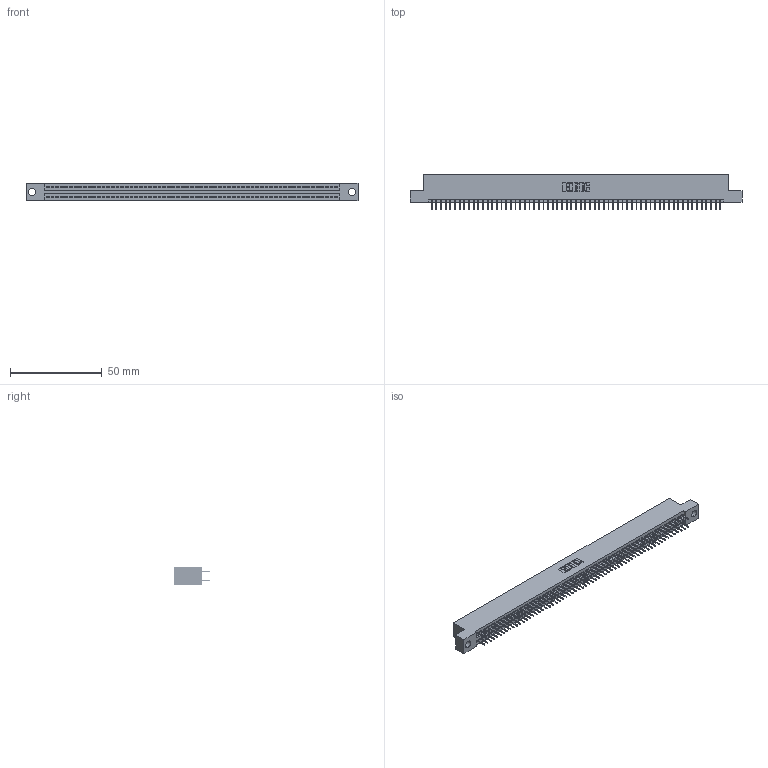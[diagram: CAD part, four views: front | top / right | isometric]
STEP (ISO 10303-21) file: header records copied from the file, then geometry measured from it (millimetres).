
FILE_DESCRIPTION (( 'STEP AP203' ), '1' );
FILE_NAME ('345-126-524-204.STEP', '2021-05-25T18:59:37', ( '' ), ( '' ), 'SwSTEP 2.0', 'SolidWorks 2020', '' );
FILE_SCHEMA (( 'CONFIG_CONTROL_DESIGN' ));
Length unit declared in the file: inch
Products named in the file (3): 345-292-001_345-293-124; 345 Part_Flush Mounting Lugs - 0.156 Dia-TI; 345-126-524-204
Assembly tree (127 placements, depth 2):
  345-126-524-204
    345 Part_Flush Mounting Lugs - 0.156 Dia-TI
    345-292-001_345-293-124  x126
Bounding box: 181.23 x 19.35 x 9.4 mm (x, y, z)
Volume: 17503.1 mm3; surface area: 25627.4 mm2
Topology: 127 solids, 127 shells, 6944 faces, 19655 edges, 12598 vertices
Faces by surface type: plane 5008, cylinder 1936
Entity records: 47097 total; most frequent: CARTESIAN_POINT 7878, ORIENTED_EDGE 7810, DIRECTION 6921, EDGE_CURVE 3905, VECTOR 3525, LINE 3525, VERTEX_POINT 2598, AXIS2_PLACEMENT_3D 1698
